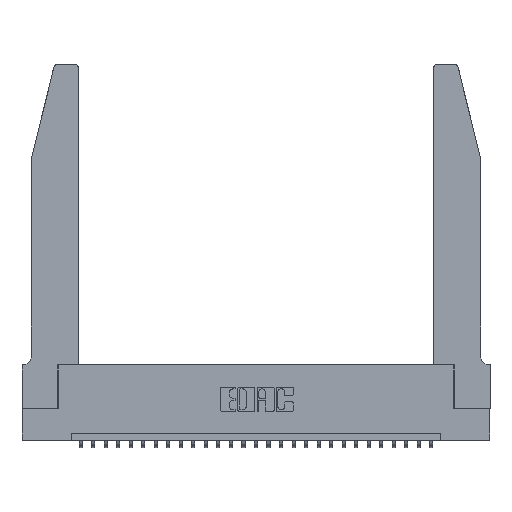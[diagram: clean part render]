
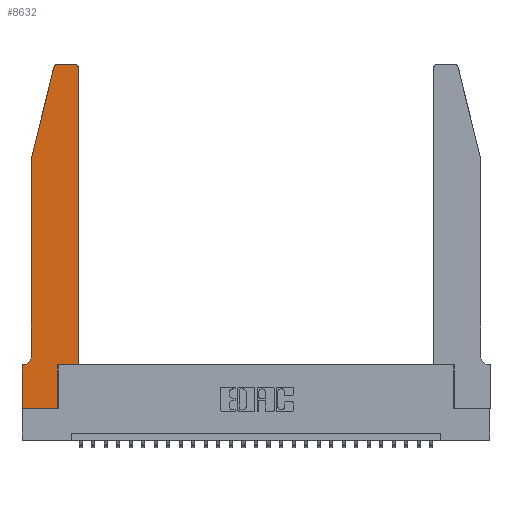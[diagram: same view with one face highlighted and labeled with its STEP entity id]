
A CAD part, top view. The second image highlights one B-rep face of the part: STEP entity #8632.
In plain terms, the highlighted planar face has unit normal (0, 0, 1).
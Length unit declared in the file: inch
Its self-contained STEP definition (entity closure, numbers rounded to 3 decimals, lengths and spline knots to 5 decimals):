
#19 = EDGE_CURVE ( 'NONE', #17027, #14389, #26092, .T. ) ;
#122 = LINE ( 'NONE', #4470, #14500 ) ;
#254 = CARTESIAN_POINT ( 'NONE',  ( 0.0755, 2., 0.37 ) ) ;
#274 = VERTEX_POINT ( 'NONE', #6422 ) ;
#732 = CARTESIAN_POINT ( 'NONE',  ( 0.4505, 2.72, 0.37 ) ) ;
#1017 = ORIENTED_EDGE ( 'NONE', *, *, #4825, .T. ) ;
#2124 = EDGE_CURVE ( 'NONE', #10597, #10709, #18404, .T. ) ;
#2340 = CARTESIAN_POINT ( 'NONE',  ( 0., 0., 0.37 ) ) ;
#2348 = VECTOR ( 'NONE', #12857, 39.37008 ) ;
#3085 = EDGE_CURVE ( 'NONE', #15742, #16326, #5312, .T. ) ;
#3298 = DIRECTION ( 'NONE',  ( -1., 0., 0. ) ) ;
#3358 = CARTESIAN_POINT ( 'NONE',  ( 0.0055, 0.42, 0.37 ) ) ;
#3581 = CARTESIAN_POINT ( 'NONE',  ( 0., 0.35, 0.37 ) ) ;
#3589 = VECTOR ( 'NONE', #17513, 39.37008 ) ;
#3639 = AXIS2_PLACEMENT_3D ( 'NONE', #11301, #6770, #26848 ) ;
#3830 = EDGE_CURVE ( 'NONE', #274, #18064, #20382, .T. ) ;
#3850 = DIRECTION ( 'NONE',  ( 0., 0., 1. ) ) ;
#3851 = CARTESIAN_POINT ( 'NONE',  ( 0.4505, 0.35, 0.37 ) ) ;
#3909 = CARTESIAN_POINT ( 'NONE',  ( 0.4205, 2.75, 0.37 ) ) ;
#4470 = CARTESIAN_POINT ( 'NONE',  ( 0.4505, 0.35, 0.37 ) ) ;
#4773 = ORIENTED_EDGE ( 'NONE', *, *, #3085, .T. ) ;
#4825 = EDGE_CURVE ( 'NONE', #16326, #10597, #13755, .T. ) ;
#5312 = LINE ( 'NONE', #254, #3589 ) ;
#6087 = ORIENTED_EDGE ( 'NONE', *, *, #28133, .T. ) ;
#6150 = CARTESIAN_POINT ( 'NONE',  ( 0.2865, 0.35, 0.37 ) ) ;
#6285 = DIRECTION ( 'NONE',  ( 0., -1., 0. ) ) ;
#6422 = CARTESIAN_POINT ( 'NONE',  ( 0.284, 2.75, 0.37 ) ) ;
#6593 = LINE ( 'NONE', #11472, #16185 ) ;
#6749 = AXIS2_PLACEMENT_3D ( 'NONE', #28326, #15151, #24409 ) ;
#6770 = DIRECTION ( 'NONE',  ( 0., 0., 1. ) ) ;
#7331 = EDGE_CURVE ( 'NONE', #25639, #28223, #19512, .T. ) ;
#8572 = VECTOR ( 'NONE', #16495, 39.37008 ) ;
#8632 = ADVANCED_FACE ( 'NONE', ( #25677 ), #13385, .T. ) ;
#9182 = ORIENTED_EDGE ( 'NONE', *, *, #22874, .T. ) ;
#10066 = DIRECTION ( 'NONE',  ( 0., 0., -1. ) ) ;
#10255 = DIRECTION ( 'NONE',  ( 0., 1., 0. ) ) ;
#10260 = CARTESIAN_POINT ( 'NONE',  ( 0.0755, 2., 0.37 ) ) ;
#10597 = VERTEX_POINT ( 'NONE', #15176 ) ;
#10709 = VERTEX_POINT ( 'NONE', #3581 ) ;
#10963 = LINE ( 'NONE', #21645, #2348 ) ;
#10994 = VECTOR ( 'NONE', #12480, 39.37008 ) ;
#11189 = DIRECTION ( 'NONE',  ( -0.239, -0.971, 0. ) ) ;
#11301 = CARTESIAN_POINT ( 'NONE',  ( 0., 0.35, 0.37 ) ) ;
#11352 = CARTESIAN_POINT ( 'NONE',  ( 0.2865, 0., 0.37 ) ) ;
#11472 = CARTESIAN_POINT ( 'NONE',  ( 0.0755, 2., 0.37 ) ) ;
#11645 = ORIENTED_EDGE ( 'NONE', *, *, #2124, .T. ) ;
#12480 = DIRECTION ( 'NONE',  ( -1., 0., 0. ) ) ;
#12620 = CIRCLE ( 'NONE', #6749, 0.03 ) ;
#12857 = DIRECTION ( 'NONE',  ( 1., 0., 0. ) ) ;
#13136 = ORIENTED_EDGE ( 'NONE', *, *, #19, .T. ) ;
#13236 = VECTOR ( 'NONE', #3298, 39.37008 ) ;
#13385 = PLANE ( 'NONE',  #3639 ) ;
#13645 = VECTOR ( 'NONE', #10255, 39.37008 ) ;
#13755 = CIRCLE ( 'NONE', #21839, 0.07 ) ;
#13757 = CARTESIAN_POINT ( 'NONE',  ( 0., 0., 0.37 ) ) ;
#14090 = CARTESIAN_POINT ( 'NONE',  ( 0.0755, 0.35, 0.37 ) ) ;
#14202 = AXIS2_PLACEMENT_3D ( 'NONE', #23562, #3850, #25842 ) ;
#14241 = CARTESIAN_POINT ( 'NONE',  ( 0.25487, 2.72718, 0.37 ) ) ;
#14389 = VERTEX_POINT ( 'NONE', #732 ) ;
#14500 = VECTOR ( 'NONE', #28389, 39.37008 ) ;
#14809 = EDGE_CURVE ( 'NONE', #21809, #25639, #10963, .T. ) ;
#15151 = DIRECTION ( 'NONE',  ( 0., 0., 1. ) ) ;
#15176 = CARTESIAN_POINT ( 'NONE',  ( 0.0055, 0.35, 0.37 ) ) ;
#15742 = VERTEX_POINT ( 'NONE', #10260 ) ;
#15891 = VERTEX_POINT ( 'NONE', #3909 ) ;
#15929 = ORIENTED_EDGE ( 'NONE', *, *, #7331, .T. ) ;
#16125 = EDGE_CURVE ( 'NONE', #18064, #15742, #6593, .T. ) ;
#16185 = VECTOR ( 'NONE', #11189, 39.37008 ) ;
#16326 = VERTEX_POINT ( 'NONE', #20877 ) ;
#16495 = DIRECTION ( 'NONE',  ( 0., 1., 0. ) ) ;
#16693 = CARTESIAN_POINT ( 'NONE',  ( 0.2605, 2.75, 0.37 ) ) ;
#17027 = VERTEX_POINT ( 'NONE', #3851 ) ;
#17513 = DIRECTION ( 'NONE',  ( 0., -1., 0. ) ) ;
#17869 = ORIENTED_EDGE ( 'NONE', *, *, #18428, .T. ) ;
#18064 = VERTEX_POINT ( 'NONE', #14241 ) ;
#18404 = LINE ( 'NONE', #14090, #13236 ) ;
#18407 = LINE ( 'NONE', #2340, #22910 ) ;
#18428 = EDGE_CURVE ( 'NONE', #14389, #15891, #12620, .T. ) ;
#19512 = LINE ( 'NONE', #21312, #13645 ) ;
#20382 = CIRCLE ( 'NONE', #14202, 0.03 ) ;
#20513 = ORIENTED_EDGE ( 'NONE', *, *, #27257, .T. ) ;
#20838 = DIRECTION ( 'NONE',  ( -1., 0., 0. ) ) ;
#20877 = CARTESIAN_POINT ( 'NONE',  ( 0.0755, 0.42, 0.37 ) ) ;
#21312 = CARTESIAN_POINT ( 'NONE',  ( 0.2865, 0.35, 0.37 ) ) ;
#21645 = CARTESIAN_POINT ( 'NONE',  ( 0., 0., 0.37 ) ) ;
#21809 = VERTEX_POINT ( 'NONE', #13757 ) ;
#21839 = AXIS2_PLACEMENT_3D ( 'NONE', #3358, #10066, #20838 ) ;
#22793 = CARTESIAN_POINT ( 'NONE',  ( 0.4505, 0.35, 0.37 ) ) ;
#22874 = EDGE_CURVE ( 'NONE', #28223, #17027, #122, .T. ) ;
#22910 = VECTOR ( 'NONE', #6285, 39.37008 ) ;
#23562 = CARTESIAN_POINT ( 'NONE',  ( 0.284, 2.72, 0.37 ) ) ;
#24409 = DIRECTION ( 'NONE',  ( 1., 0., 0. ) ) ;
#25639 = VERTEX_POINT ( 'NONE', #11352 ) ;
#25665 = ORIENTED_EDGE ( 'NONE', *, *, #3830, .T. ) ;
#25677 = FACE_OUTER_BOUND ( 'NONE', #26556, .T. ) ;
#25842 = DIRECTION ( 'NONE',  ( 1., 0., 0. ) ) ;
#26092 = LINE ( 'NONE', #22793, #8572 ) ;
#26556 = EDGE_LOOP ( 'NONE', ( #6087, #25665, #27446, #4773, #1017, #11645, #20513, #26694, #15929, #9182, #13136, #17869 ) ) ;
#26694 = ORIENTED_EDGE ( 'NONE', *, *, #14809, .T. ) ;
#26848 = DIRECTION ( 'NONE',  ( 1., 0., 0. ) ) ;
#27257 = EDGE_CURVE ( 'NONE', #10709, #21809, #18407, .T. ) ;
#27446 = ORIENTED_EDGE ( 'NONE', *, *, #16125, .T. ) ;
#27792 = LINE ( 'NONE', #16693, #10994 ) ;
#28133 = EDGE_CURVE ( 'NONE', #15891, #274, #27792, .T. ) ;
#28223 = VERTEX_POINT ( 'NONE', #6150 ) ;
#28326 = CARTESIAN_POINT ( 'NONE',  ( 0.4205, 2.72, 0.37 ) ) ;
#28389 = DIRECTION ( 'NONE',  ( 1., 0., 0. ) ) ;
